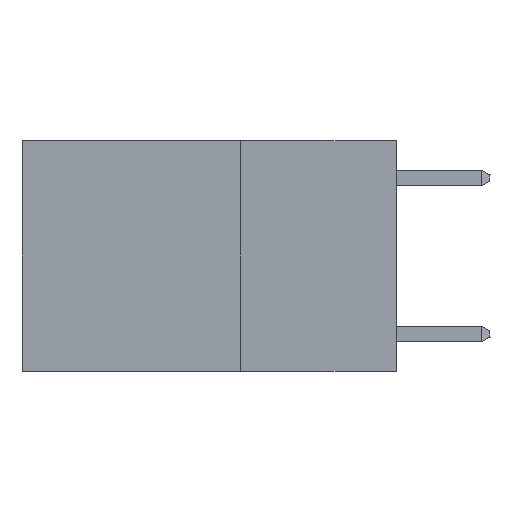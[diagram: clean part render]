
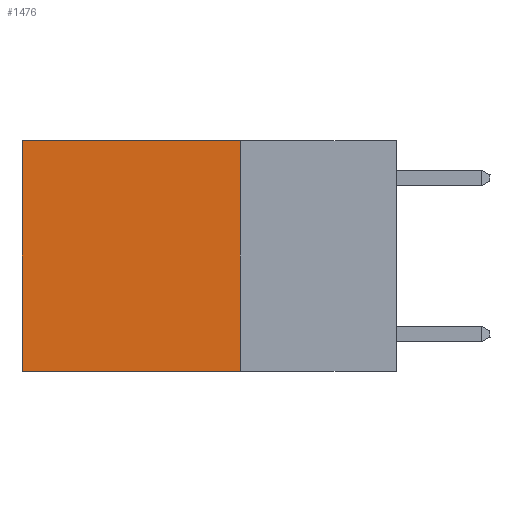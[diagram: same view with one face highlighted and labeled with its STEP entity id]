
A CAD part, left-side view. The second image highlights one B-rep face of the part: STEP entity #1476.
In plain terms, the highlighted planar face has unit normal (-1, 0, 0).
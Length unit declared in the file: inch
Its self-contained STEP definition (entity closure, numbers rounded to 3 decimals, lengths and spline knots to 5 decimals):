
#148 = DIRECTION ( 'NONE',  ( 1., 0., 0. ) ) ;
#274 = VECTOR ( 'NONE', #11400, 39.37008 ) ;
#426 = CARTESIAN_POINT ( 'NONE',  ( 0.2625, 0.25, 0. ) ) ;
#454 = ORIENTED_EDGE ( 'NONE', *, *, #1710, .T. ) ;
#462 = CARTESIAN_POINT ( 'NONE',  ( 0.2625, 0.6, 0. ) ) ;
#1476 = ADVANCED_FACE ( 'NONE', ( #18469 ), #20234, .F. ) ;
#1710 = EDGE_CURVE ( 'NONE', #6993, #20380, #15128, .T. ) ;
#2019 = ORIENTED_EDGE ( 'NONE', *, *, #14807, .F. ) ;
#4172 = CARTESIAN_POINT ( 'NONE',  ( 0.2625, 0.25, 0. ) ) ;
#4288 = ORIENTED_EDGE ( 'NONE', *, *, #8628, .F. ) ;
#4974 = VECTOR ( 'NONE', #12682, 39.37008 ) ;
#5962 = EDGE_CURVE ( 'NONE', #9628, #6993, #18989, .T. ) ;
#6218 = VECTOR ( 'NONE', #6794, 39.37008 ) ;
#6792 = ORIENTED_EDGE ( 'NONE', *, *, #5962, .T. ) ;
#6794 = DIRECTION ( 'NONE',  ( 0., 1., 0. ) ) ;
#6993 = VERTEX_POINT ( 'NONE', #7061 ) ;
#7061 = CARTESIAN_POINT ( 'NONE',  ( 0.2625, 0.6, 0. ) ) ;
#7302 = AXIS2_PLACEMENT_3D ( 'NONE', #4172, #148, #9556 ) ;
#8628 = EDGE_CURVE ( 'NONE', #9628, #17913, #19878, .T. ) ;
#9556 = DIRECTION ( 'NONE',  ( 0., 0., -1. ) ) ;
#9628 = VERTEX_POINT ( 'NONE', #426 ) ;
#9962 = CARTESIAN_POINT ( 'NONE',  ( 0.2625, 0.25, 0. ) ) ;
#10841 = CARTESIAN_POINT ( 'NONE',  ( 0.2625, 0.25, -0.37 ) ) ;
#11400 = DIRECTION ( 'NONE',  ( 0., 1., 0. ) ) ;
#12421 = CARTESIAN_POINT ( 'NONE',  ( 0.2625, 0.25, -0.37 ) ) ;
#12537 = EDGE_LOOP ( 'NONE', ( #454, #2019, #4288, #6792 ) ) ;
#12682 = DIRECTION ( 'NONE',  ( 0., 0., -1. ) ) ;
#14789 = DIRECTION ( 'NONE',  ( 0., 0., -1. ) ) ;
#14807 = EDGE_CURVE ( 'NONE', #17913, #20380, #21865, .T. ) ;
#15128 = LINE ( 'NONE', #462, #19664 ) ;
#17437 = CARTESIAN_POINT ( 'NONE',  ( 0.2625, 0.25, 0. ) ) ;
#17913 = VERTEX_POINT ( 'NONE', #12421 ) ;
#18469 = FACE_OUTER_BOUND ( 'NONE', #12537, .T. ) ;
#18989 = LINE ( 'NONE', #17437, #6218 ) ;
#19664 = VECTOR ( 'NONE', #14789, 39.37008 ) ;
#19878 = LINE ( 'NONE', #9962, #4974 ) ;
#20234 = PLANE ( 'NONE',  #7302 ) ;
#20243 = CARTESIAN_POINT ( 'NONE',  ( 0.2625, 0.6, -0.37 ) ) ;
#20380 = VERTEX_POINT ( 'NONE', #20243 ) ;
#21865 = LINE ( 'NONE', #10841, #274 ) ;
